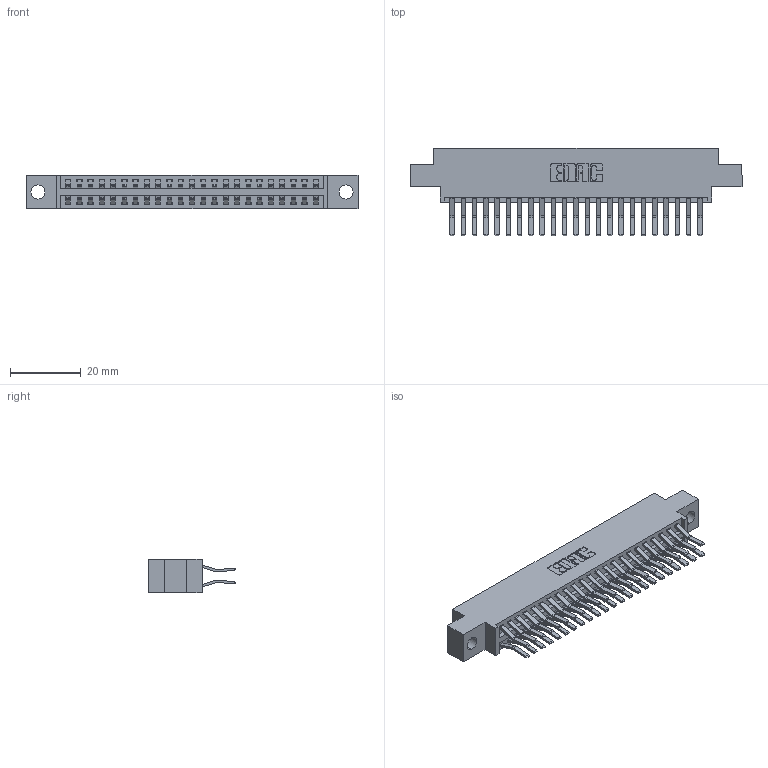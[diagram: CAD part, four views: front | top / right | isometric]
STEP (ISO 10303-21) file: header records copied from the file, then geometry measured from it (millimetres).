
FILE_DESCRIPTION (( 'STEP AP203' ), '1' );
FILE_NAME ('346-046-560-804.STEP', '2022-05-20T20:46:57', ( '' ), ( '' ), 'SwSTEP 2.0', 'SolidWorks 2020', '' );
FILE_SCHEMA (( 'CONFIG_CONTROL_DESIGN' ));
Length unit declared in the file: inch
Products named in the file (3): 346 Part_0.170 Offset - 0.156 Dia-TH; 346-046-560-804; 345-292-001_560 Tail
Assembly tree (47 placements, depth 2):
  346-046-560-804
    346 Part_0.170 Offset - 0.156 Dia-TH
    345-292-001_560 Tail  x46
Bounding box: 93.6 x 24.78 x 9.4 mm (x, y, z)
Volume: 9020.4 mm3; surface area: 12932.5 mm2
Topology: 47 solids, 47 shells, 2624 faces, 7783 edges, 5126 vertices
Faces by surface type: plane 1704, cylinder 920
Entity records: 18207 total; most frequent: CARTESIAN_POINT 3034, ORIENTED_EDGE 2966, DIRECTION 2727, EDGE_CURVE 1483, LINE 1255, VECTOR 1255, VERTEX_POINT 986, AXIS2_PLACEMENT_3D 736
